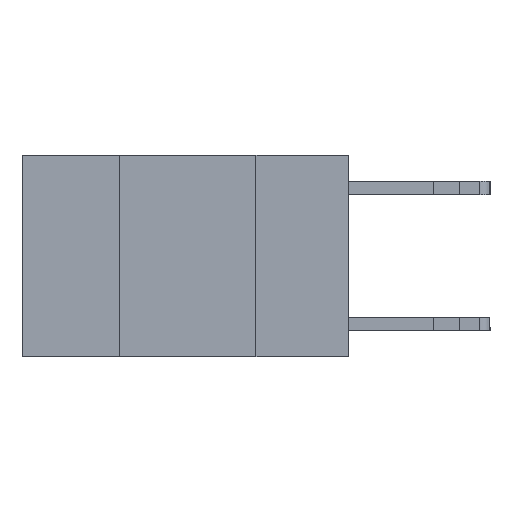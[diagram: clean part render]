
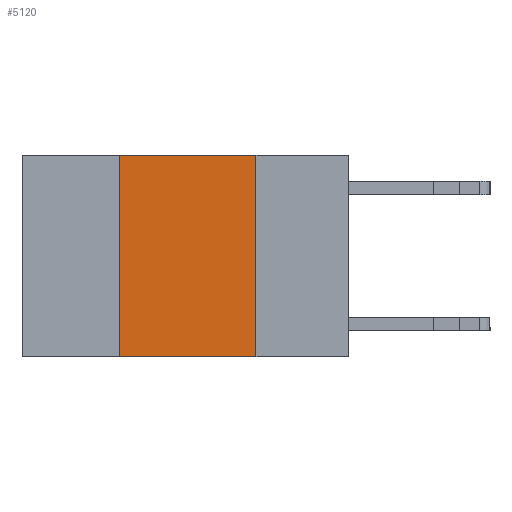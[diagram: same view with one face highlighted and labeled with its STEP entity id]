
A CAD part, left-side view. The second image highlights one B-rep face of the part: STEP entity #5120.
In plain terms, the highlighted planar face has unit normal (-1, 0, 0).
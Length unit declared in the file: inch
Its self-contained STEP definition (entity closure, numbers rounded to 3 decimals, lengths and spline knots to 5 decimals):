
#2750 = VERTEX_POINT ( 'NONE', #5063 ) ;
#3543 = ORIENTED_EDGE ( 'NONE', *, *, #20516, .F. ) ;
#3560 = CARTESIAN_POINT ( 'NONE',  ( 0., 0.42, 0. ) ) ;
#4089 = CARTESIAN_POINT ( 'NONE',  ( 0., 0.17, -0.37 ) ) ;
#4839 = CARTESIAN_POINT ( 'NONE',  ( 0., 0.17, 0. ) ) ;
#5063 = CARTESIAN_POINT ( 'NONE',  ( 0., 0.17, 0. ) ) ;
#5120 = ADVANCED_FACE ( 'NONE', ( #13426 ), #15366, .F. ) ;
#5481 = VECTOR ( 'NONE', #21777, 39.37008 ) ;
#5514 = VERTEX_POINT ( 'NONE', #17837 ) ;
#6916 = VERTEX_POINT ( 'NONE', #4089 ) ;
#7789 = EDGE_CURVE ( 'NONE', #15980, #2750, #22227, .T. ) ;
#8325 = DIRECTION ( 'NONE',  ( 0., -1., 0. ) ) ;
#8947 = LINE ( 'NONE', #20510, #21612 ) ;
#10227 = LINE ( 'NONE', #3560, #5481 ) ;
#11473 = DIRECTION ( 'NONE',  ( 0., -1., 0. ) ) ;
#12997 = CARTESIAN_POINT ( 'NONE',  ( 0., 0.6, 0. ) ) ;
#13139 = DIRECTION ( 'NONE',  ( 1., 0., 0. ) ) ;
#13426 = FACE_OUTER_BOUND ( 'NONE', #13476, .T. ) ;
#13476 = EDGE_LOOP ( 'NONE', ( #22199, #27493, #3543, #23220 ) ) ;
#14548 = VECTOR ( 'NONE', #20845, 39.37008 ) ;
#15366 = PLANE ( 'NONE',  #16436 ) ;
#15980 = VERTEX_POINT ( 'NONE', #18278 ) ;
#16436 = AXIS2_PLACEMENT_3D ( 'NONE', #12997, #13139, #28820 ) ;
#17837 = CARTESIAN_POINT ( 'NONE',  ( 0., 0.42, -0.37 ) ) ;
#18278 = CARTESIAN_POINT ( 'NONE',  ( 0., 0.42, 0. ) ) ;
#20252 = LINE ( 'NONE', #4839, #14548 ) ;
#20510 = CARTESIAN_POINT ( 'NONE',  ( 0., 0.6, -0.37 ) ) ;
#20516 = EDGE_CURVE ( 'NONE', #5514, #15980, #10227, .T. ) ;
#20845 = DIRECTION ( 'NONE',  ( 0., 0., -1. ) ) ;
#21155 = EDGE_CURVE ( 'NONE', #5514, #6916, #8947, .T. ) ;
#21612 = VECTOR ( 'NONE', #11473, 39.37008 ) ;
#21777 = DIRECTION ( 'NONE',  ( 0., 0., 1. ) ) ;
#22199 = ORIENTED_EDGE ( 'NONE', *, *, #22738, .F. ) ;
#22227 = LINE ( 'NONE', #28572, #23617 ) ;
#22738 = EDGE_CURVE ( 'NONE', #2750, #6916, #20252, .T. ) ;
#23220 = ORIENTED_EDGE ( 'NONE', *, *, #21155, .T. ) ;
#23617 = VECTOR ( 'NONE', #8325, 39.37008 ) ;
#27493 = ORIENTED_EDGE ( 'NONE', *, *, #7789, .F. ) ;
#28572 = CARTESIAN_POINT ( 'NONE',  ( 0., 0.6, 0. ) ) ;
#28820 = DIRECTION ( 'NONE',  ( 0., 0., -1. ) ) ;
